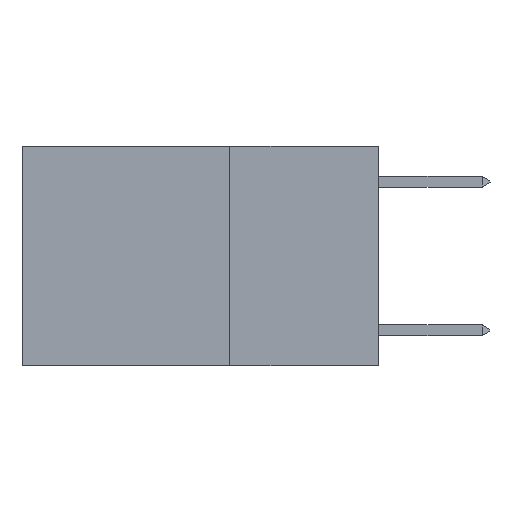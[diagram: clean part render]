
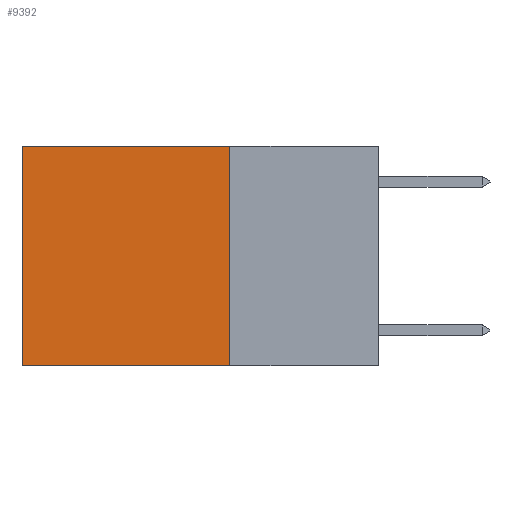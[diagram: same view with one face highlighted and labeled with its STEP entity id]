
A CAD part, left-side view. The second image highlights one B-rep face of the part: STEP entity #9392.
In plain terms, the highlighted planar face has unit normal (-1, 0, 0).
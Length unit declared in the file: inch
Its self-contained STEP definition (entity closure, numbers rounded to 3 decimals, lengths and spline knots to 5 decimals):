
#152 = VECTOR ( 'NONE', #9970, 39.37008 ) ;
#429 = ORIENTED_EDGE ( 'NONE', *, *, #1910, .F. ) ;
#609 = DIRECTION ( 'NONE',  ( 0., 1., 0. ) ) ;
#670 = VERTEX_POINT ( 'NONE', #10070 ) ;
#692 = DIRECTION ( 'NONE',  ( 1., 0., 0. ) ) ;
#704 = DIRECTION ( 'NONE',  ( 0., 1., 0. ) ) ;
#1028 = EDGE_CURVE ( 'NONE', #670, #4113, #1038, .T. ) ;
#1038 = LINE ( 'NONE', #1130, #2465 ) ;
#1130 = CARTESIAN_POINT ( 'NONE',  ( 0.2625, 0.6, 0. ) ) ;
#1594 = FACE_OUTER_BOUND ( 'NONE', #5235, .T. ) ;
#1910 = EDGE_CURVE ( 'NONE', #6149, #4113, #4451, .T. ) ;
#2284 = LINE ( 'NONE', #8681, #8656 ) ;
#2465 = VECTOR ( 'NONE', #8165, 39.37008 ) ;
#3011 = CARTESIAN_POINT ( 'NONE',  ( 0.2625, 0.6, -0.37 ) ) ;
#3649 = VECTOR ( 'NONE', #609, 39.37008 ) ;
#4113 = VERTEX_POINT ( 'NONE', #3011 ) ;
#4451 = LINE ( 'NONE', #8428, #3649 ) ;
#4596 = CARTESIAN_POINT ( 'NONE',  ( 0.2625, 0.25, 0. ) ) ;
#4961 = PLANE ( 'NONE',  #7562 ) ;
#5192 = CARTESIAN_POINT ( 'NONE',  ( 0.2625, 0.25, 0. ) ) ;
#5235 = EDGE_LOOP ( 'NONE', ( #9718, #429, #7590, #7335 ) ) ;
#6149 = VERTEX_POINT ( 'NONE', #7568 ) ;
#6881 = EDGE_CURVE ( 'NONE', #8725, #6149, #7480, .T. ) ;
#7195 = CARTESIAN_POINT ( 'NONE',  ( 0.2625, 0.25, 0. ) ) ;
#7255 = DIRECTION ( 'NONE',  ( 0., 0., -1. ) ) ;
#7335 = ORIENTED_EDGE ( 'NONE', *, *, #8685, .T. ) ;
#7480 = LINE ( 'NONE', #5192, #152 ) ;
#7562 = AXIS2_PLACEMENT_3D ( 'NONE', #7195, #692, #7255 ) ;
#7568 = CARTESIAN_POINT ( 'NONE',  ( 0.2625, 0.25, -0.37 ) ) ;
#7590 = ORIENTED_EDGE ( 'NONE', *, *, #6881, .F. ) ;
#8165 = DIRECTION ( 'NONE',  ( 0., 0., -1. ) ) ;
#8428 = CARTESIAN_POINT ( 'NONE',  ( 0.2625, 0.25, -0.37 ) ) ;
#8656 = VECTOR ( 'NONE', #704, 39.37008 ) ;
#8681 = CARTESIAN_POINT ( 'NONE',  ( 0.2625, 0.25, 0. ) ) ;
#8685 = EDGE_CURVE ( 'NONE', #8725, #670, #2284, .T. ) ;
#8725 = VERTEX_POINT ( 'NONE', #4596 ) ;
#9392 = ADVANCED_FACE ( 'NONE', ( #1594 ), #4961, .F. ) ;
#9718 = ORIENTED_EDGE ( 'NONE', *, *, #1028, .T. ) ;
#9970 = DIRECTION ( 'NONE',  ( 0., 0., -1. ) ) ;
#10070 = CARTESIAN_POINT ( 'NONE',  ( 0.2625, 0.6, 0. ) ) ;
